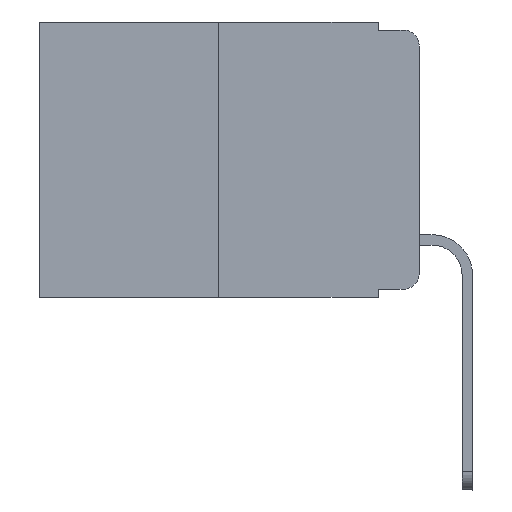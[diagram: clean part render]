
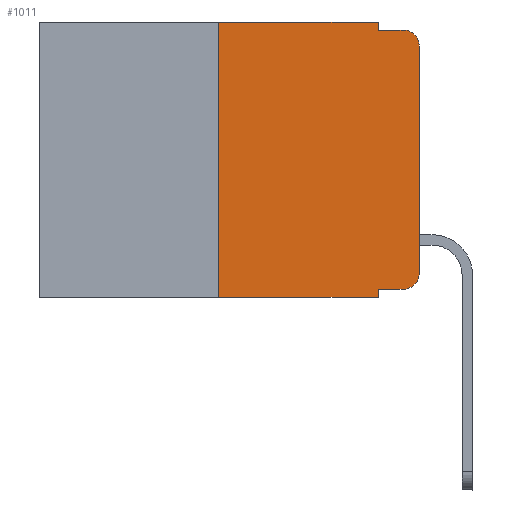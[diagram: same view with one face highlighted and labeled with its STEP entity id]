
A CAD part, left-side view. The second image highlights one B-rep face of the part: STEP entity #1011.
In plain terms, the highlighted planar face has unit normal (-1, 0, 0).
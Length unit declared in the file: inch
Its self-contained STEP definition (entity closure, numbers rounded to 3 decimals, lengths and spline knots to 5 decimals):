
#81 = CARTESIAN_POINT ( 'NONE',  ( 0., 0.051, 0. ) ) ;
#117 = VERTEX_POINT ( 'NONE', #16540 ) ;
#123 = VERTEX_POINT ( 'NONE', #6500 ) ;
#180 = LINE ( 'NONE', #8673, #15697 ) ;
#536 = DIRECTION ( 'NONE',  ( 0., 0., -1. ) ) ;
#1004 = LINE ( 'NONE', #18216, #15177 ) ;
#1011 = ADVANCED_FACE ( 'NONE', ( #2969 ), #5596, .F. ) ;
#1567 = DIRECTION ( 'NONE',  ( 0., 0., -1. ) ) ;
#2014 = DIRECTION ( 'NONE',  ( -1., 0., 0. ) ) ;
#2193 = VERTEX_POINT ( 'NONE', #16688 ) ;
#2573 = EDGE_CURVE ( 'NONE', #123, #7774, #1004, .T. ) ;
#2839 = VERTEX_POINT ( 'NONE', #14935 ) ;
#2969 = FACE_OUTER_BOUND ( 'NONE', #6270, .T. ) ;
#3502 = VECTOR ( 'NONE', #16459, 39.37008 ) ;
#3721 = EDGE_CURVE ( 'NONE', #117, #16461, #10755, .T. ) ;
#3978 = EDGE_CURVE ( 'NONE', #2193, #123, #15985, .T. ) ;
#4187 = DIRECTION ( 'NONE',  ( 0., -1., 0. ) ) ;
#4554 = VECTOR ( 'NONE', #9592, 39.37008 ) ;
#4783 = CARTESIAN_POINT ( 'NONE',  ( 0., 0., 0. ) ) ;
#4937 = CARTESIAN_POINT ( 'NONE',  ( 0., 0.051, 0. ) ) ;
#4940 = DIRECTION ( 'NONE',  ( 0., 0., -1. ) ) ;
#5317 = CARTESIAN_POINT ( 'NONE',  ( 0., 0.25, -0.343 ) ) ;
#5415 = VERTEX_POINT ( 'NONE', #8376 ) ;
#5520 = LINE ( 'NONE', #11250, #9250 ) ;
#5596 = PLANE ( 'NONE',  #13721 ) ;
#5610 = EDGE_CURVE ( 'NONE', #117, #17895, #5755, .T. ) ;
#5755 = LINE ( 'NONE', #11494, #11273 ) ;
#5787 = CARTESIAN_POINT ( 'NONE',  ( 0., 0.473, 0. ) ) ;
#6256 = CARTESIAN_POINT ( 'NONE',  ( 0., 0.25, 0. ) ) ;
#6270 = EDGE_LOOP ( 'NONE', ( #11576, #9003, #10762, #9203, #15353, #8865, #15655, #16823, #7533, #11367 ) ) ;
#6500 = CARTESIAN_POINT ( 'NONE',  ( 0., 0.051, -0.01 ) ) ;
#6591 = EDGE_CURVE ( 'NONE', #5415, #7774, #10198, .T. ) ;
#7533 = ORIENTED_EDGE ( 'NONE', *, *, #5610, .T. ) ;
#7663 = CARTESIAN_POINT ( 'NONE',  ( 0., 0.02, -0.03 ) ) ;
#7774 = VERTEX_POINT ( 'NONE', #9658 ) ;
#8196 = DIRECTION ( 'NONE',  ( 0., -1., 0. ) ) ;
#8200 = EDGE_CURVE ( 'NONE', #14614, #9693, #5520, .T. ) ;
#8207 = VECTOR ( 'NONE', #10423, 39.37008 ) ;
#8376 = CARTESIAN_POINT ( 'NONE',  ( 0., 0., -0.03 ) ) ;
#8503 = DIRECTION ( 'NONE',  ( 1., 0., 0. ) ) ;
#8673 = CARTESIAN_POINT ( 'NONE',  ( 0., 0.473, 0. ) ) ;
#8865 = ORIENTED_EDGE ( 'NONE', *, *, #8200, .F. ) ;
#8977 = AXIS2_PLACEMENT_3D ( 'NONE', #7663, #12097, #4940 ) ;
#9003 = ORIENTED_EDGE ( 'NONE', *, *, #6591, .T. ) ;
#9203 = ORIENTED_EDGE ( 'NONE', *, *, #3978, .F. ) ;
#9250 = VECTOR ( 'NONE', #16945, 39.37008 ) ;
#9402 = LINE ( 'NONE', #16713, #4554 ) ;
#9592 = DIRECTION ( 'NONE',  ( 0., -1., 0. ) ) ;
#9658 = CARTESIAN_POINT ( 'NONE',  ( 0., 0.02, -0.01 ) ) ;
#9693 = VERTEX_POINT ( 'NONE', #6256 ) ;
#10026 = CARTESIAN_POINT ( 'NONE',  ( 0., 0.02, -0.313 ) ) ;
#10198 = CIRCLE ( 'NONE', #8977, 0.02 ) ;
#10423 = DIRECTION ( 'NONE',  ( 0., 0., 1. ) ) ;
#10755 = LINE ( 'NONE', #4937, #3502 ) ;
#10762 = ORIENTED_EDGE ( 'NONE', *, *, #2573, .F. ) ;
#10987 = VECTOR ( 'NONE', #1567, 39.37008 ) ;
#10988 = EDGE_CURVE ( 'NONE', #2839, #5415, #17522, .T. ) ;
#11127 = CARTESIAN_POINT ( 'NONE',  ( 0., 0.051, -0.343 ) ) ;
#11250 = CARTESIAN_POINT ( 'NONE',  ( 0., 0.25, 0. ) ) ;
#11273 = VECTOR ( 'NONE', #17184, 39.37008 ) ;
#11367 = ORIENTED_EDGE ( 'NONE', *, *, #17991, .T. ) ;
#11494 = CARTESIAN_POINT ( 'NONE',  ( 0., 0.051, -0.333 ) ) ;
#11576 = ORIENTED_EDGE ( 'NONE', *, *, #10988, .T. ) ;
#12097 = DIRECTION ( 'NONE',  ( -1., 0., 0. ) ) ;
#12167 = CARTESIAN_POINT ( 'NONE',  ( 0., 0.02, -0.333 ) ) ;
#12180 = EDGE_CURVE ( 'NONE', #9693, #2193, #180, .T. ) ;
#13563 = CIRCLE ( 'NONE', #15049, 0.02 ) ;
#13721 = AXIS2_PLACEMENT_3D ( 'NONE', #5787, #8503, #15814 ) ;
#14614 = VERTEX_POINT ( 'NONE', #5317 ) ;
#14935 = CARTESIAN_POINT ( 'NONE',  ( 0., 0., -0.313 ) ) ;
#15049 = AXIS2_PLACEMENT_3D ( 'NONE', #10026, #2014, #536 ) ;
#15177 = VECTOR ( 'NONE', #8196, 39.37008 ) ;
#15353 = ORIENTED_EDGE ( 'NONE', *, *, #12180, .F. ) ;
#15655 = ORIENTED_EDGE ( 'NONE', *, *, #16840, .T. ) ;
#15697 = VECTOR ( 'NONE', #4187, 39.37008 ) ;
#15814 = DIRECTION ( 'NONE',  ( 0., 0., -1. ) ) ;
#15985 = LINE ( 'NONE', #81, #10987 ) ;
#16459 = DIRECTION ( 'NONE',  ( 0., 0., -1. ) ) ;
#16461 = VERTEX_POINT ( 'NONE', #11127 ) ;
#16540 = CARTESIAN_POINT ( 'NONE',  ( 0., 0.051, -0.333 ) ) ;
#16688 = CARTESIAN_POINT ( 'NONE',  ( 0., 0.051, 0. ) ) ;
#16713 = CARTESIAN_POINT ( 'NONE',  ( 0., 0.473, -0.343 ) ) ;
#16823 = ORIENTED_EDGE ( 'NONE', *, *, #3721, .F. ) ;
#16840 = EDGE_CURVE ( 'NONE', #14614, #16461, #9402, .T. ) ;
#16945 = DIRECTION ( 'NONE',  ( 0., 0., 1. ) ) ;
#17184 = DIRECTION ( 'NONE',  ( 0., -1., 0. ) ) ;
#17522 = LINE ( 'NONE', #4783, #8207 ) ;
#17895 = VERTEX_POINT ( 'NONE', #12167 ) ;
#17991 = EDGE_CURVE ( 'NONE', #17895, #2839, #13563, .T. ) ;
#18216 = CARTESIAN_POINT ( 'NONE',  ( 0., 0.051, -0.01 ) ) ;
